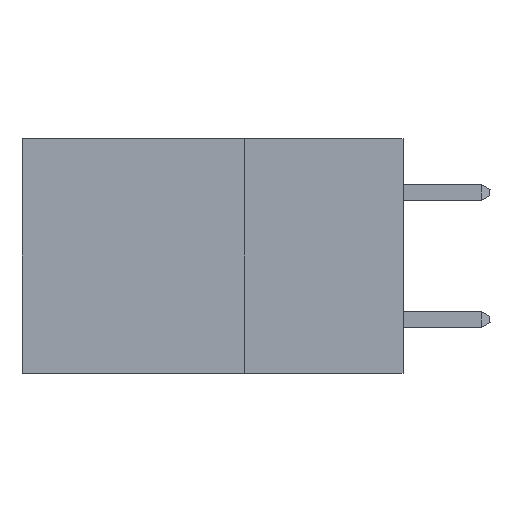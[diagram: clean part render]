
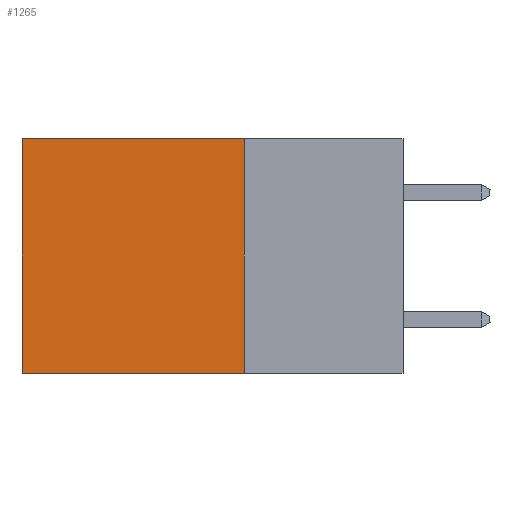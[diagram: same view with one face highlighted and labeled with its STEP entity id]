
A CAD part, left-side view. The second image highlights one B-rep face of the part: STEP entity #1265.
In plain terms, the highlighted planar face has unit normal (-1, 0, 0).
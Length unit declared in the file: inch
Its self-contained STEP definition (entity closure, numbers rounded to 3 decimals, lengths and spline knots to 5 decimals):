
#218 = ORIENTED_EDGE ( 'NONE', *, *, #13438, .F. ) ;
#1265 = ADVANCED_FACE ( 'NONE', ( #36184 ), #9342, .F. ) ;
#2818 = LINE ( 'NONE', #24271, #5236 ) ;
#3639 = EDGE_CURVE ( 'NONE', #10275, #37462, #36933, .T. ) ;
#3779 = DIRECTION ( 'NONE',  ( 0., 0., -1. ) ) ;
#5236 = VECTOR ( 'NONE', #30346, 39.37008 ) ;
#6271 = CARTESIAN_POINT ( 'NONE',  ( 0.2875, 0.25, 0. ) ) ;
#7169 = CARTESIAN_POINT ( 'NONE',  ( 0.2875, 0.6, 0. ) ) ;
#7320 = ORIENTED_EDGE ( 'NONE', *, *, #3639, .F. ) ;
#7629 = LINE ( 'NONE', #27083, #30742 ) ;
#8043 = DIRECTION ( 'NONE',  ( 0., 1., 0. ) ) ;
#8443 = ORIENTED_EDGE ( 'NONE', *, *, #30061, .T. ) ;
#9342 = PLANE ( 'NONE',  #40295 ) ;
#9479 = DIRECTION ( 'NONE',  ( 0., 0., -1. ) ) ;
#10275 = VERTEX_POINT ( 'NONE', #34353 ) ;
#12133 = ORIENTED_EDGE ( 'NONE', *, *, #31216, .T. ) ;
#13438 = EDGE_CURVE ( 'NONE', #37462, #21807, #7629, .T. ) ;
#14356 = CARTESIAN_POINT ( 'NONE',  ( 0.2875, 0.25, -0.37 ) ) ;
#14631 = DIRECTION ( 'NONE',  ( 0., 1., 0. ) ) ;
#21807 = VERTEX_POINT ( 'NONE', #28796 ) ;
#24271 = CARTESIAN_POINT ( 'NONE',  ( 0.2875, 0.6, 0. ) ) ;
#25871 = CARTESIAN_POINT ( 'NONE',  ( 0.2875, 0.25, 0. ) ) ;
#27043 = VECTOR ( 'NONE', #8043, 39.37008 ) ;
#27083 = CARTESIAN_POINT ( 'NONE',  ( 0.2875, 0.25, -0.37 ) ) ;
#28300 = DIRECTION ( 'NONE',  ( 1., 0., 0. ) ) ;
#28623 = VECTOR ( 'NONE', #3779, 39.37008 ) ;
#28796 = CARTESIAN_POINT ( 'NONE',  ( 0.2875, 0.6, -0.37 ) ) ;
#30030 = CARTESIAN_POINT ( 'NONE',  ( 0.2875, 0.25, 0. ) ) ;
#30061 = EDGE_CURVE ( 'NONE', #10275, #40086, #35323, .T. ) ;
#30346 = DIRECTION ( 'NONE',  ( 0., 0., -1. ) ) ;
#30742 = VECTOR ( 'NONE', #14631, 39.37008 ) ;
#31216 = EDGE_CURVE ( 'NONE', #40086, #21807, #2818, .T. ) ;
#34353 = CARTESIAN_POINT ( 'NONE',  ( 0.2875, 0.25, 0. ) ) ;
#35323 = LINE ( 'NONE', #30030, #27043 ) ;
#36184 = FACE_OUTER_BOUND ( 'NONE', #39765, .T. ) ;
#36933 = LINE ( 'NONE', #25871, #28623 ) ;
#37462 = VERTEX_POINT ( 'NONE', #14356 ) ;
#39765 = EDGE_LOOP ( 'NONE', ( #12133, #218, #7320, #8443 ) ) ;
#40086 = VERTEX_POINT ( 'NONE', #7169 ) ;
#40295 = AXIS2_PLACEMENT_3D ( 'NONE', #6271, #28300, #9479 ) ;
